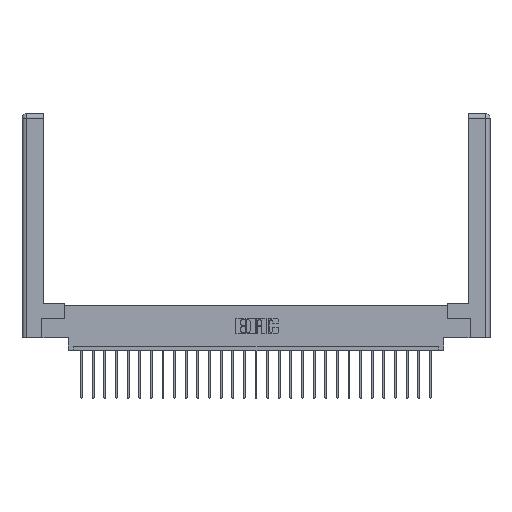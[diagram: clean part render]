
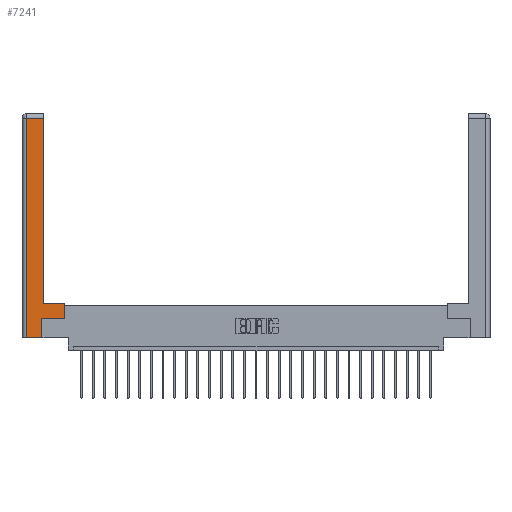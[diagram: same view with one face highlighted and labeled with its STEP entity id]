
A CAD part, top view. The second image highlights one B-rep face of the part: STEP entity #7241.
In plain terms, the highlighted planar face has unit normal (0, 0, 1).
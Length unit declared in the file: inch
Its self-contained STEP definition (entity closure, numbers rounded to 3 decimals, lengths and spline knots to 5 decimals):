
#191 = VECTOR ( 'NONE', #7070, 39.37008 ) ;
#581 = VECTOR ( 'NONE', #3823, 39.37008 ) ;
#1689 = AXIS2_PLACEMENT_3D ( 'NONE', #3821, #16213, #14470 ) ;
#1955 = EDGE_CURVE ( 'NONE', #4845, #5576, #17145, .T. ) ;
#2286 = ORIENTED_EDGE ( 'NONE', *, *, #26661, .T. ) ;
#2739 = VERTEX_POINT ( 'NONE', #15958 ) ;
#2743 = ORIENTED_EDGE ( 'NONE', *, *, #21618, .T. ) ;
#2770 = CARTESIAN_POINT ( 'NONE',  ( 0.295, 0.45, 0. ) ) ;
#2907 = EDGE_CURVE ( 'NONE', #15754, #2739, #15506, .T. ) ;
#3177 = ORIENTED_EDGE ( 'NONE', *, *, #2907, .T. ) ;
#3290 = DIRECTION ( 'NONE',  ( 0., -1., 0. ) ) ;
#3821 = CARTESIAN_POINT ( 'NONE',  ( 0., 0., 0. ) ) ;
#3823 = DIRECTION ( 'NONE',  ( -1., 0., 0. ) ) ;
#4781 = DIRECTION ( 'NONE',  ( 0., 1., 0. ) ) ;
#4820 = DIRECTION ( 'NONE',  ( 0., 1., 0. ) ) ;
#4845 = VERTEX_POINT ( 'NONE', #22151 ) ;
#5111 = LINE ( 'NONE', #21767, #23866 ) ;
#5312 = VECTOR ( 'NONE', #3290, 39.37008 ) ;
#5576 = VERTEX_POINT ( 'NONE', #11103 ) ;
#5670 = ORIENTED_EDGE ( 'NONE', *, *, #25899, .T. ) ;
#6473 = EDGE_CURVE ( 'NONE', #15041, #14316, #7420, .T. ) ;
#6502 = CARTESIAN_POINT ( 'NONE',  ( 0.295, 0.45, 0. ) ) ;
#7070 = DIRECTION ( 'NONE',  ( -1., 0., 0. ) ) ;
#7241 = ADVANCED_FACE ( 'NONE', ( #23175 ), #22642, .F. ) ;
#7261 = LINE ( 'NONE', #23400, #26355 ) ;
#7420 = LINE ( 'NONE', #22550, #19909 ) ;
#10260 = VECTOR ( 'NONE', #4820, 39.37008 ) ;
#11103 = CARTESIAN_POINT ( 'NONE',  ( 0.0615, 0., 0. ) ) ;
#12683 = LINE ( 'NONE', #2770, #191 ) ;
#14316 = VERTEX_POINT ( 'NONE', #18524 ) ;
#14470 = DIRECTION ( 'NONE',  ( -1., 0., 0. ) ) ;
#14582 = CARTESIAN_POINT ( 'NONE',  ( 0.295, 3., 0. ) ) ;
#15041 = VERTEX_POINT ( 'NONE', #16838 ) ;
#15506 = LINE ( 'NONE', #14582, #24707 ) ;
#15754 = VERTEX_POINT ( 'NONE', #6502 ) ;
#15958 = CARTESIAN_POINT ( 'NONE',  ( 0.295, 2.94, 0. ) ) ;
#16213 = DIRECTION ( 'NONE',  ( 0., 0., -1. ) ) ;
#16214 = EDGE_CURVE ( 'NONE', #5576, #18735, #7261, .T. ) ;
#16621 = ORIENTED_EDGE ( 'NONE', *, *, #1955, .T. ) ;
#16838 = CARTESIAN_POINT ( 'NONE',  ( 0.265, 0.245, 0. ) ) ;
#17145 = LINE ( 'NONE', #26637, #5312 ) ;
#17247 = EDGE_LOOP ( 'NONE', ( #3177, #22089, #16621, #25559, #2743, #22641, #2286, #5670 ) ) ;
#17716 = CARTESIAN_POINT ( 'NONE',  ( 0.565, 0.45, 0. ) ) ;
#18405 = DIRECTION ( 'NONE',  ( 1., 0., 0. ) ) ;
#18524 = CARTESIAN_POINT ( 'NONE',  ( 0.565, 0.245, 0. ) ) ;
#18735 = VERTEX_POINT ( 'NONE', #25769 ) ;
#19909 = VECTOR ( 'NONE', #18405, 39.37008 ) ;
#21618 = EDGE_CURVE ( 'NONE', #18735, #15041, #23100, .T. ) ;
#21767 = CARTESIAN_POINT ( 'NONE',  ( 0.565, 0.45, 0. ) ) ;
#22089 = ORIENTED_EDGE ( 'NONE', *, *, #25208, .T. ) ;
#22151 = CARTESIAN_POINT ( 'NONE',  ( 0.0615, 2.94, 0. ) ) ;
#22550 = CARTESIAN_POINT ( 'NONE',  ( 0.565, 0.245, 0. ) ) ;
#22607 = LINE ( 'NONE', #26901, #581 ) ;
#22641 = ORIENTED_EDGE ( 'NONE', *, *, #6473, .T. ) ;
#22642 = PLANE ( 'NONE',  #1689 ) ;
#22752 = DIRECTION ( 'NONE',  ( 0., 1., 0. ) ) ;
#23100 = LINE ( 'NONE', #26035, #10260 ) ;
#23175 = FACE_OUTER_BOUND ( 'NONE', #17247, .T. ) ;
#23400 = CARTESIAN_POINT ( 'NONE',  ( 0.265, 0., 0. ) ) ;
#23681 = VERTEX_POINT ( 'NONE', #17716 ) ;
#23866 = VECTOR ( 'NONE', #4781, 39.37008 ) ;
#24707 = VECTOR ( 'NONE', #22752, 39.37008 ) ;
#25208 = EDGE_CURVE ( 'NONE', #2739, #4845, #22607, .T. ) ;
#25423 = DIRECTION ( 'NONE',  ( 1., 0., 0. ) ) ;
#25559 = ORIENTED_EDGE ( 'NONE', *, *, #16214, .T. ) ;
#25769 = CARTESIAN_POINT ( 'NONE',  ( 0.265, 0., 0. ) ) ;
#25899 = EDGE_CURVE ( 'NONE', #23681, #15754, #12683, .T. ) ;
#26035 = CARTESIAN_POINT ( 'NONE',  ( 0.265, 0.245, 0. ) ) ;
#26355 = VECTOR ( 'NONE', #25423, 39.37008 ) ;
#26637 = CARTESIAN_POINT ( 'NONE',  ( 0.0615, 0., 0. ) ) ;
#26661 = EDGE_CURVE ( 'NONE', #14316, #23681, #5111, .T. ) ;
#26901 = CARTESIAN_POINT ( 'NONE',  ( 0.0615, 2.94, 0. ) ) ;
